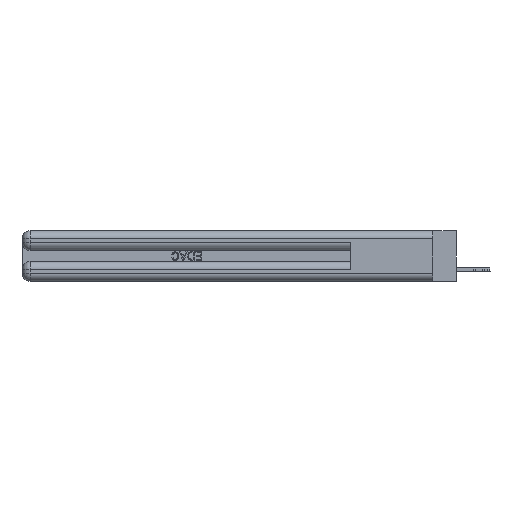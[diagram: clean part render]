
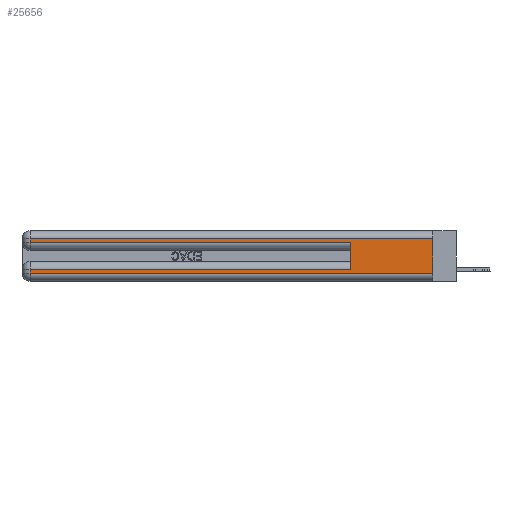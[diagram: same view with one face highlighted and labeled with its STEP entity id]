
A CAD part, left-side view. The second image highlights one B-rep face of the part: STEP entity #25656.
In plain terms, the highlighted planar face has unit normal (-1, 0, 0).
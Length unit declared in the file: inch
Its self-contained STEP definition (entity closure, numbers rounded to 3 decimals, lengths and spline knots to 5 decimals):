
#129 = VERTEX_POINT ( 'NONE', #4687 ) ;
#1286 = EDGE_CURVE ( 'NONE', #32380, #19791, #7970, .T. ) ;
#2000 = ORIENTED_EDGE ( 'NONE', *, *, #2113, .T. ) ;
#2113 = EDGE_CURVE ( 'NONE', #13165, #32380, #29538, .T. ) ;
#2134 = VECTOR ( 'NONE', #13535, 39.37008 ) ;
#2348 = VECTOR ( 'NONE', #35673, 39.37008 ) ;
#3563 = CARTESIAN_POINT ( 'NONE',  ( 0., 0., 0.085 ) ) ;
#3824 = ORIENTED_EDGE ( 'NONE', *, *, #1286, .T. ) ;
#4687 = CARTESIAN_POINT ( 'NONE',  ( 0., 0.6, 0.285 ) ) ;
#5170 = DIRECTION ( 'NONE',  ( 0., 0., -1. ) ) ;
#5190 = EDGE_CURVE ( 'NONE', #43069, #129, #37121, .T. ) ;
#5314 = CARTESIAN_POINT ( 'NONE',  ( 0., 2.94, 0.31 ) ) ;
#5999 = ORIENTED_EDGE ( 'NONE', *, *, #27558, .F. ) ;
#7297 = DIRECTION ( 'NONE',  ( 0., 0., 1. ) ) ;
#7970 = LINE ( 'NONE', #25337, #42237 ) ;
#8179 = LINE ( 'NONE', #17433, #24009 ) ;
#8428 = ORIENTED_EDGE ( 'NONE', *, *, #5190, .T. ) ;
#8561 = CARTESIAN_POINT ( 'NONE',  ( 0., 0., 0.31 ) ) ;
#8575 = EDGE_CURVE ( 'NONE', #31932, #14703, #25462, .T. ) ;
#9237 = CARTESIAN_POINT ( 'NONE',  ( 0., 0., 0.06 ) ) ;
#11616 = ORIENTED_EDGE ( 'NONE', *, *, #8575, .T. ) ;
#12335 = LINE ( 'NONE', #15643, #2348 ) ;
#13165 = VERTEX_POINT ( 'NONE', #43517 ) ;
#13535 = DIRECTION ( 'NONE',  ( 0., 1., 0. ) ) ;
#13690 = ORIENTED_EDGE ( 'NONE', *, *, #27824, .T. ) ;
#13716 = DIRECTION ( 'NONE',  ( 0., 0., -1. ) ) ;
#14703 = VERTEX_POINT ( 'NONE', #5314 ) ;
#15123 = CARTESIAN_POINT ( 'NONE',  ( 0., 2.94, 0.285 ) ) ;
#15198 = DIRECTION ( 'NONE',  ( 0., -1., 0. ) ) ;
#15643 = CARTESIAN_POINT ( 'NONE',  ( 0., 0., 0.37 ) ) ;
#16595 = VECTOR ( 'NONE', #15198, 39.37008 ) ;
#17350 = EDGE_CURVE ( 'NONE', #31932, #22473, #12335, .T. ) ;
#17433 = CARTESIAN_POINT ( 'NONE',  ( 0., 0.6, 0.145 ) ) ;
#17491 = ORIENTED_EDGE ( 'NONE', *, *, #17350, .F. ) ;
#17591 = CARTESIAN_POINT ( 'NONE',  ( 0., 0., 0.31 ) ) ;
#19306 = DIRECTION ( 'NONE',  ( 0., 0., -1. ) ) ;
#19791 = VERTEX_POINT ( 'NONE', #32327 ) ;
#21054 = AXIS2_PLACEMENT_3D ( 'NONE', #30806, #34213, #13716 ) ;
#22101 = DIRECTION ( 'NONE',  ( 0., 1., 0. ) ) ;
#22473 = VERTEX_POINT ( 'NONE', #9237 ) ;
#24009 = VECTOR ( 'NONE', #7297, 39.37008 ) ;
#25337 = CARTESIAN_POINT ( 'NONE',  ( 0., 2.94, 0.37 ) ) ;
#25462 = LINE ( 'NONE', #8561, #41309 ) ;
#25656 = ADVANCED_FACE ( 'NONE', ( #28351 ), #26987, .F. ) ;
#26076 = CARTESIAN_POINT ( 'NONE',  ( 0., 0., 0.06 ) ) ;
#26987 = PLANE ( 'NONE',  #21054 ) ;
#27558 = EDGE_CURVE ( 'NONE', #13165, #129, #8179, .T. ) ;
#27824 = EDGE_CURVE ( 'NONE', #19791, #22473, #36072, .T. ) ;
#28246 = EDGE_LOOP ( 'NONE', ( #17491, #11616, #33212, #8428, #5999, #2000, #3824, #13690 ) ) ;
#28351 = FACE_OUTER_BOUND ( 'NONE', #28246, .T. ) ;
#29538 = LINE ( 'NONE', #3563, #2134 ) ;
#30806 = CARTESIAN_POINT ( 'NONE',  ( 0., 0., 0.37 ) ) ;
#31932 = VERTEX_POINT ( 'NONE', #17591 ) ;
#32101 = LINE ( 'NONE', #39501, #35258 ) ;
#32327 = CARTESIAN_POINT ( 'NONE',  ( 0., 2.94, 0.06 ) ) ;
#32380 = VERTEX_POINT ( 'NONE', #33743 ) ;
#33212 = ORIENTED_EDGE ( 'NONE', *, *, #35586, .T. ) ;
#33743 = CARTESIAN_POINT ( 'NONE',  ( 0., 2.94, 0.085 ) ) ;
#34213 = DIRECTION ( 'NONE',  ( 1., 0., 0. ) ) ;
#35258 = VECTOR ( 'NONE', #19306, 39.37008 ) ;
#35586 = EDGE_CURVE ( 'NONE', #14703, #43069, #32101, .T. ) ;
#35673 = DIRECTION ( 'NONE',  ( 0., 0., -1. ) ) ;
#35959 = DIRECTION ( 'NONE',  ( 0., -1., 0. ) ) ;
#35984 = CARTESIAN_POINT ( 'NONE',  ( 0., 0., 0.285 ) ) ;
#36072 = LINE ( 'NONE', #26076, #38215 ) ;
#37121 = LINE ( 'NONE', #35984, #16595 ) ;
#38215 = VECTOR ( 'NONE', #35959, 39.37008 ) ;
#39501 = CARTESIAN_POINT ( 'NONE',  ( 0., 2.94, 0.37 ) ) ;
#41309 = VECTOR ( 'NONE', #22101, 39.37008 ) ;
#42237 = VECTOR ( 'NONE', #5170, 39.37008 ) ;
#43069 = VERTEX_POINT ( 'NONE', #15123 ) ;
#43517 = CARTESIAN_POINT ( 'NONE',  ( 0., 0.6, 0.085 ) ) ;
